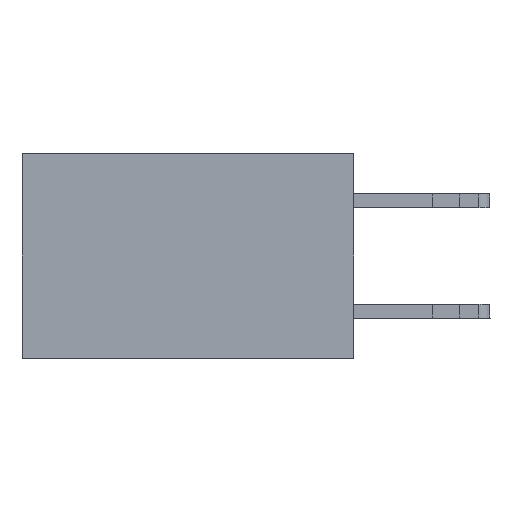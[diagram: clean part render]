
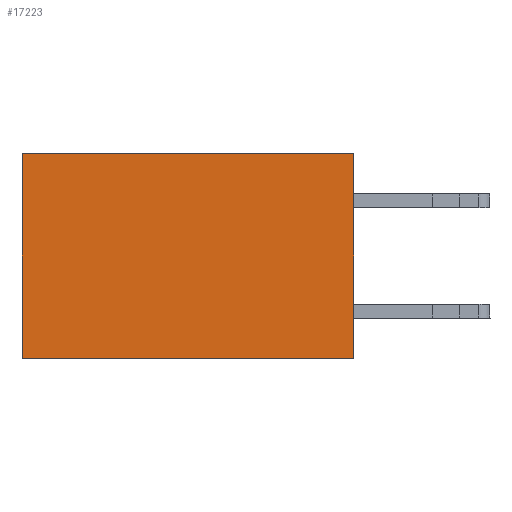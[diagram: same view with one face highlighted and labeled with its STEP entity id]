
A CAD part, left-side view. The second image highlights one B-rep face of the part: STEP entity #17223.
In plain terms, the highlighted planar face has unit normal (-1, 0, 0).
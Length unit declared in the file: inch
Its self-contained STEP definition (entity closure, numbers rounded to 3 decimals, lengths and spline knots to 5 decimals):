
#434 = CARTESIAN_POINT ( 'NONE',  ( 0.2875, 0.6, 0. ) ) ;
#1262 = VECTOR ( 'NONE', #18330, 39.37008 ) ;
#1997 = FACE_OUTER_BOUND ( 'NONE', #3549, .T. ) ;
#2587 = EDGE_CURVE ( 'NONE', #6960, #2952, #5331, .T. ) ;
#2952 = VERTEX_POINT ( 'NONE', #6792 ) ;
#2970 = ORIENTED_EDGE ( 'NONE', *, *, #2587, .F. ) ;
#3549 = EDGE_LOOP ( 'NONE', ( #8312, #16840, #2970, #16635 ) ) ;
#3826 = LINE ( 'NONE', #434, #12069 ) ;
#4703 = CARTESIAN_POINT ( 'NONE',  ( 0.2875, 0., 0. ) ) ;
#4759 = CARTESIAN_POINT ( 'NONE',  ( 0.2875, 0.6, 0. ) ) ;
#5331 = LINE ( 'NONE', #4703, #1262 ) ;
#5427 = PLANE ( 'NONE',  #10786 ) ;
#5887 = EDGE_CURVE ( 'NONE', #6960, #6861, #15342, .T. ) ;
#6640 = CARTESIAN_POINT ( 'NONE',  ( 0.2875, 0., 0. ) ) ;
#6792 = CARTESIAN_POINT ( 'NONE',  ( 0.2875, 0., -0.37 ) ) ;
#6861 = VERTEX_POINT ( 'NONE', #4759 ) ;
#6960 = VERTEX_POINT ( 'NONE', #11141 ) ;
#8312 = ORIENTED_EDGE ( 'NONE', *, *, #12078, .T. ) ;
#8601 = DIRECTION ( 'NONE',  ( 0., 0., -1. ) ) ;
#9900 = VERTEX_POINT ( 'NONE', #14980 ) ;
#10786 = AXIS2_PLACEMENT_3D ( 'NONE', #16169, #17591, #8601 ) ;
#11141 = CARTESIAN_POINT ( 'NONE',  ( 0.2875, 0., 0. ) ) ;
#11285 = VECTOR ( 'NONE', #18683, 39.37008 ) ;
#12069 = VECTOR ( 'NONE', #12853, 39.37008 ) ;
#12078 = EDGE_CURVE ( 'NONE', #6861, #9900, #3826, .T. ) ;
#12853 = DIRECTION ( 'NONE',  ( 0., 0., -1. ) ) ;
#14510 = VECTOR ( 'NONE', #17856, 39.37008 ) ;
#14980 = CARTESIAN_POINT ( 'NONE',  ( 0.2875, 0.6, -0.37 ) ) ;
#15342 = LINE ( 'NONE', #6640, #11285 ) ;
#16169 = CARTESIAN_POINT ( 'NONE',  ( 0.2875, 0., 0. ) ) ;
#16635 = ORIENTED_EDGE ( 'NONE', *, *, #5887, .T. ) ;
#16840 = ORIENTED_EDGE ( 'NONE', *, *, #18217, .F. ) ;
#17223 = ADVANCED_FACE ( 'NONE', ( #1997 ), #5427, .F. ) ;
#17591 = DIRECTION ( 'NONE',  ( 1., 0., 0. ) ) ;
#17856 = DIRECTION ( 'NONE',  ( 0., 1., 0. ) ) ;
#17872 = LINE ( 'NONE', #19248, #14510 ) ;
#18217 = EDGE_CURVE ( 'NONE', #2952, #9900, #17872, .T. ) ;
#18330 = DIRECTION ( 'NONE',  ( 0., 0., -1. ) ) ;
#18683 = DIRECTION ( 'NONE',  ( 0., 1., 0. ) ) ;
#19248 = CARTESIAN_POINT ( 'NONE',  ( 0.2875, 0., -0.37 ) ) ;
